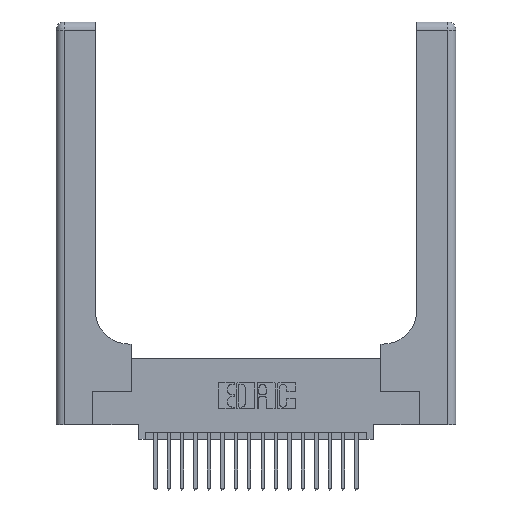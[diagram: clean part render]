
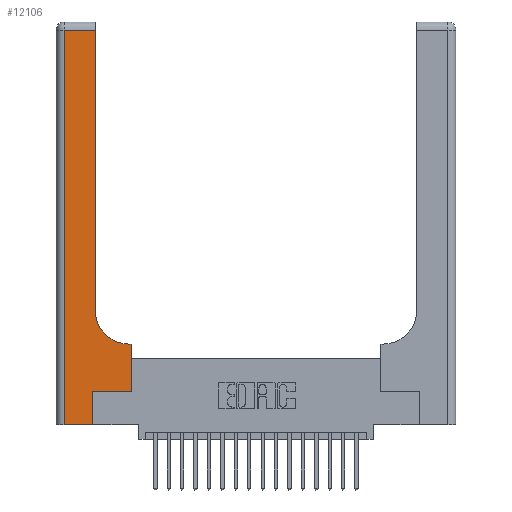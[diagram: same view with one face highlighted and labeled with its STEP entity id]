
A CAD part, top view. The second image highlights one B-rep face of the part: STEP entity #12106.
In plain terms, the highlighted planar face has unit normal (0, 0, 1).
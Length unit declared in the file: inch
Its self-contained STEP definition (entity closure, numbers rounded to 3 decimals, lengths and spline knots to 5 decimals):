
#58 = VERTEX_POINT ( 'NONE', #20455 ) ;
#288 = EDGE_CURVE ( 'NONE', #3244, #12459, #21070, .T. ) ;
#1054 = ORIENTED_EDGE ( 'NONE', *, *, #6055, .T. ) ;
#1225 = VECTOR ( 'NONE', #5994, 39.37008 ) ;
#1272 = VERTEX_POINT ( 'NONE', #1548 ) ;
#1548 = CARTESIAN_POINT ( 'NONE',  ( 0.5415, 0.6, 0.37 ) ) ;
#1650 = VECTOR ( 'NONE', #5018, 39.37008 ) ;
#1925 = ORIENTED_EDGE ( 'NONE', *, *, #6537, .T. ) ;
#2214 = CARTESIAN_POINT ( 'NONE',  ( 0.2915, 2.94, 0.37 ) ) ;
#2641 = CARTESIAN_POINT ( 'NONE',  ( 0., 0., 0.37 ) ) ;
#3124 = ORIENTED_EDGE ( 'NONE', *, *, #16326, .T. ) ;
#3208 = VERTEX_POINT ( 'NONE', #15375 ) ;
#3244 = VERTEX_POINT ( 'NONE', #13788 ) ;
#3551 = EDGE_CURVE ( 'NONE', #12459, #11703, #10546, .T. ) ;
#3570 = VECTOR ( 'NONE', #17016, 39.37008 ) ;
#4091 = DIRECTION ( 'NONE',  ( 0., 0., -1. ) ) ;
#4612 = ORIENTED_EDGE ( 'NONE', *, *, #288, .T. ) ;
#4726 = VECTOR ( 'NONE', #6121, 39.37008 ) ;
#5018 = DIRECTION ( 'NONE',  ( -1., 0., 0. ) ) ;
#5577 = CARTESIAN_POINT ( 'NONE',  ( 0.2915, 0.6, 0.37 ) ) ;
#5994 = DIRECTION ( 'NONE',  ( 0., 1., 0. ) ) ;
#6055 = EDGE_CURVE ( 'NONE', #19957, #58, #20893, .T. ) ;
#6099 = DIRECTION ( 'NONE',  ( 1., 0., 0. ) ) ;
#6121 = DIRECTION ( 'NONE',  ( 0., -1., 0. ) ) ;
#6512 = EDGE_CURVE ( 'NONE', #11378, #1272, #9919, .T. ) ;
#6537 = EDGE_CURVE ( 'NONE', #1272, #3244, #12735, .T. ) ;
#6813 = CARTESIAN_POINT ( 'NONE',  ( 0.06, 0., 0.37 ) ) ;
#6913 = CARTESIAN_POINT ( 'NONE',  ( 0.269, 0.25, 0.37 ) ) ;
#6930 = ORIENTED_EDGE ( 'NONE', *, *, #18652, .T. ) ;
#7025 = CARTESIAN_POINT ( 'NONE',  ( 0.06, 2.94, 0.37 ) ) ;
#7164 = CARTESIAN_POINT ( 'NONE',  ( 0.269, 0., 0.37 ) ) ;
#7797 = CARTESIAN_POINT ( 'NONE',  ( 0.06, 3., 0.37 ) ) ;
#8251 = CARTESIAN_POINT ( 'NONE',  ( 0., 3., 0.37 ) ) ;
#8802 = VECTOR ( 'NONE', #19902, 39.37008 ) ;
#8834 = DIRECTION ( 'NONE',  ( 0., 1., 0. ) ) ;
#8877 = VECTOR ( 'NONE', #15531, 39.37008 ) ;
#9919 = LINE ( 'NONE', #5577, #8877 ) ;
#10546 = LINE ( 'NONE', #16579, #1650 ) ;
#11212 = CARTESIAN_POINT ( 'NONE',  ( 0.5585, 0.6, 0.37 ) ) ;
#11378 = VERTEX_POINT ( 'NONE', #11212 ) ;
#11560 = DIRECTION ( 'NONE',  ( -1., 0., 0. ) ) ;
#11703 = VERTEX_POINT ( 'NONE', #7025 ) ;
#12106 = ADVANCED_FACE ( 'NONE', ( #17955 ), #18073, .F. ) ;
#12238 = VECTOR ( 'NONE', #6099, 39.37008 ) ;
#12459 = VERTEX_POINT ( 'NONE', #2214 ) ;
#12735 = CIRCLE ( 'NONE', #14229, 0.25 ) ;
#13157 = LINE ( 'NONE', #6913, #8802 ) ;
#13225 = LINE ( 'NONE', #7164, #21376 ) ;
#13554 = LINE ( 'NONE', #7797, #4726 ) ;
#13788 = CARTESIAN_POINT ( 'NONE',  ( 0.2915, 0.85, 0.37 ) ) ;
#14020 = CARTESIAN_POINT ( 'NONE',  ( 0.5415, 0.85, 0.37 ) ) ;
#14229 = AXIS2_PLACEMENT_3D ( 'NONE', #14020, #4091, #15677 ) ;
#14832 = AXIS2_PLACEMENT_3D ( 'NONE', #8251, #21311, #11560 ) ;
#15064 = EDGE_LOOP ( 'NONE', ( #4612, #16088, #3124, #1054, #18829, #18955, #6930, #15346, #1925 ) ) ;
#15346 = ORIENTED_EDGE ( 'NONE', *, *, #6512, .T. ) ;
#15375 = CARTESIAN_POINT ( 'NONE',  ( 0.269, 0.25, 0.37 ) ) ;
#15488 = EDGE_CURVE ( 'NONE', #58, #3208, #13225, .T. ) ;
#15531 = DIRECTION ( 'NONE',  ( -1., 0., 0. ) ) ;
#15677 = DIRECTION ( 'NONE',  ( 1., 0., 0. ) ) ;
#16088 = ORIENTED_EDGE ( 'NONE', *, *, #3551, .T. ) ;
#16326 = EDGE_CURVE ( 'NONE', #11703, #19957, #13554, .T. ) ;
#16579 = CARTESIAN_POINT ( 'NONE',  ( 0., 2.94, 0.37 ) ) ;
#16813 = CARTESIAN_POINT ( 'NONE',  ( 0.5585, 0.25, 0.37 ) ) ;
#17016 = DIRECTION ( 'NONE',  ( 0., 1., 0. ) ) ;
#17070 = CARTESIAN_POINT ( 'NONE',  ( 0.2915, 3., 0.37 ) ) ;
#17807 = VERTEX_POINT ( 'NONE', #16813 ) ;
#17955 = FACE_OUTER_BOUND ( 'NONE', #15064, .T. ) ;
#18073 = PLANE ( 'NONE',  #14832 ) ;
#18652 = EDGE_CURVE ( 'NONE', #17807, #11378, #18827, .T. ) ;
#18827 = LINE ( 'NONE', #19165, #1225 ) ;
#18829 = ORIENTED_EDGE ( 'NONE', *, *, #15488, .T. ) ;
#18955 = ORIENTED_EDGE ( 'NONE', *, *, #19430, .T. ) ;
#19165 = CARTESIAN_POINT ( 'NONE',  ( 0.5585, 0.25, 0.37 ) ) ;
#19430 = EDGE_CURVE ( 'NONE', #3208, #17807, #13157, .T. ) ;
#19902 = DIRECTION ( 'NONE',  ( 1., 0., 0. ) ) ;
#19957 = VERTEX_POINT ( 'NONE', #6813 ) ;
#20455 = CARTESIAN_POINT ( 'NONE',  ( 0.269, 0., 0.37 ) ) ;
#20893 = LINE ( 'NONE', #2641, #12238 ) ;
#21070 = LINE ( 'NONE', #17070, #3570 ) ;
#21311 = DIRECTION ( 'NONE',  ( 0., 0., -1. ) ) ;
#21376 = VECTOR ( 'NONE', #8834, 39.37008 ) ;
